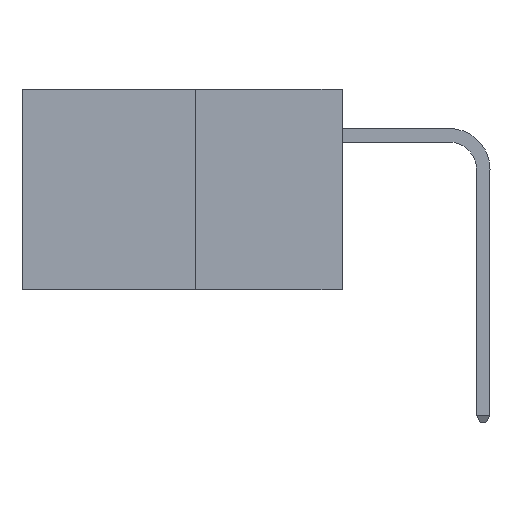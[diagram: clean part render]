
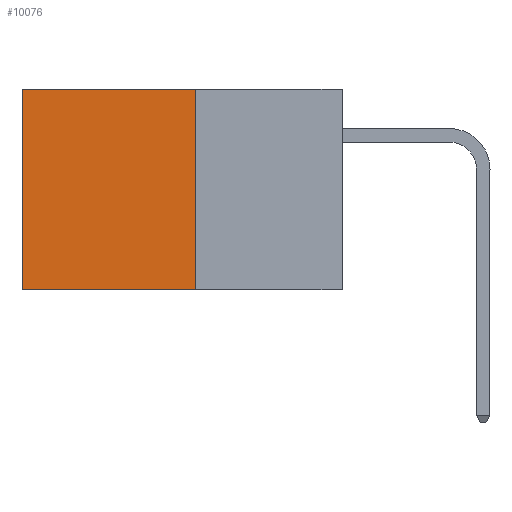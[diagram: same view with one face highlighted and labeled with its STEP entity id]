
A CAD part, left-side view. The second image highlights one B-rep face of the part: STEP entity #10076.
In plain terms, the highlighted planar face has unit normal (-1, 0, 0).
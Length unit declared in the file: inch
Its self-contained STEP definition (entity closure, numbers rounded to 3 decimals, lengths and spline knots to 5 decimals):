
#108 = LINE ( 'NONE', #3296, #10630 ) ;
#131 = DIRECTION ( 'NONE',  ( 1., 0., 0. ) ) ;
#295 = CARTESIAN_POINT ( 'NONE',  ( 0.277, 0.59, -0.37 ) ) ;
#537 = VECTOR ( 'NONE', #10381, 39.37008 ) ;
#1103 = EDGE_CURVE ( 'NONE', #4078, #6992, #108, .T. ) ;
#1271 = CARTESIAN_POINT ( 'NONE',  ( 0.277, 0.27, -0.37 ) ) ;
#1546 = FACE_OUTER_BOUND ( 'NONE', #12777, .T. ) ;
#2012 = DIRECTION ( 'NONE',  ( 0., 0., -1. ) ) ;
#2939 = CARTESIAN_POINT ( 'NONE',  ( 0.277, 0.59, 0. ) ) ;
#3296 = CARTESIAN_POINT ( 'NONE',  ( 0.277, 0.59, -0.37 ) ) ;
#3709 = CARTESIAN_POINT ( 'NONE',  ( 0.277, 0.27, 0. ) ) ;
#3944 = LINE ( 'NONE', #1271, #537 ) ;
#4074 = ORIENTED_EDGE ( 'NONE', *, *, #11289, .F. ) ;
#4078 = VERTEX_POINT ( 'NONE', #2939 ) ;
#4142 = DIRECTION ( 'NONE',  ( 0., 1., 0. ) ) ;
#4546 = CARTESIAN_POINT ( 'NONE',  ( 0.277, 0.27, -0.37 ) ) ;
#5036 = ORIENTED_EDGE ( 'NONE', *, *, #10120, .F. ) ;
#5756 = VERTEX_POINT ( 'NONE', #11094 ) ;
#6317 = PLANE ( 'NONE',  #12674 ) ;
#6992 = VERTEX_POINT ( 'NONE', #295 ) ;
#7244 = EDGE_CURVE ( 'NONE', #5756, #4078, #8506, .T. ) ;
#7312 = DIRECTION ( 'NONE',  ( 0., 0., -1. ) ) ;
#7975 = VERTEX_POINT ( 'NONE', #4546 ) ;
#8506 = LINE ( 'NONE', #3709, #13105 ) ;
#8556 = DIRECTION ( 'NONE',  ( 0., 1., 0. ) ) ;
#9302 = VECTOR ( 'NONE', #8556, 39.37008 ) ;
#9337 = CARTESIAN_POINT ( 'NONE',  ( 0.277, 0.27, -0.37 ) ) ;
#9588 = LINE ( 'NONE', #11482, #9302 ) ;
#10076 = ADVANCED_FACE ( 'NONE', ( #1546 ), #6317, .F. ) ;
#10120 = EDGE_CURVE ( 'NONE', #5756, #7975, #3944, .T. ) ;
#10381 = DIRECTION ( 'NONE',  ( 0., 0., -1. ) ) ;
#10630 = VECTOR ( 'NONE', #2012, 39.37008 ) ;
#10681 = ORIENTED_EDGE ( 'NONE', *, *, #7244, .T. ) ;
#11094 = CARTESIAN_POINT ( 'NONE',  ( 0.277, 0.27, 0. ) ) ;
#11289 = EDGE_CURVE ( 'NONE', #7975, #6992, #9588, .T. ) ;
#11482 = CARTESIAN_POINT ( 'NONE',  ( 0.277, 0.27, -0.37 ) ) ;
#12661 = ORIENTED_EDGE ( 'NONE', *, *, #1103, .T. ) ;
#12674 = AXIS2_PLACEMENT_3D ( 'NONE', #9337, #131, #7312 ) ;
#12777 = EDGE_LOOP ( 'NONE', ( #12661, #4074, #5036, #10681 ) ) ;
#13105 = VECTOR ( 'NONE', #4142, 39.37008 ) ;
